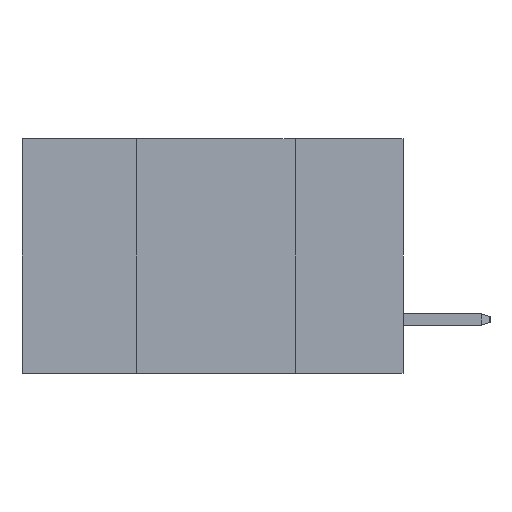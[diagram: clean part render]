
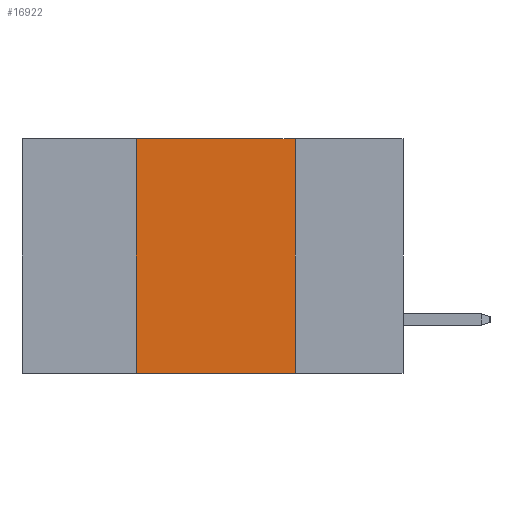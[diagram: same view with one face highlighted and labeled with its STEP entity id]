
A CAD part, left-side view. The second image highlights one B-rep face of the part: STEP entity #16922.
In plain terms, the highlighted planar face has unit normal (-1, 0, 0).
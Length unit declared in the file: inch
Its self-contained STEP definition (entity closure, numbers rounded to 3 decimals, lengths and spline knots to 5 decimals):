
#703 = CARTESIAN_POINT ( 'NONE',  ( 0., 0.42, -0.37 ) ) ;
#1049 = LINE ( 'NONE', #22835, #8461 ) ;
#1106 = LINE ( 'NONE', #4960, #2140 ) ;
#1616 = EDGE_CURVE ( 'NONE', #22002, #8231, #1049, .T. ) ;
#2140 = VECTOR ( 'NONE', #11341, 39.37008 ) ;
#2306 = ORIENTED_EDGE ( 'NONE', *, *, #1616, .F. ) ;
#2631 = EDGE_CURVE ( 'NONE', #6597, #22002, #1106, .T. ) ;
#3078 = VECTOR ( 'NONE', #9740, 39.37008 ) ;
#3267 = CARTESIAN_POINT ( 'NONE',  ( 0., 0.42, 0. ) ) ;
#4795 = ORIENTED_EDGE ( 'NONE', *, *, #22974, .T. ) ;
#4960 = CARTESIAN_POINT ( 'NONE',  ( 0., 0.6, 0. ) ) ;
#5110 = VECTOR ( 'NONE', #12046, 39.37008 ) ;
#5680 = PLANE ( 'NONE',  #6244 ) ;
#6244 = AXIS2_PLACEMENT_3D ( 'NONE', #11934, #25717, #17767 ) ;
#6597 = VERTEX_POINT ( 'NONE', #3267 ) ;
#7059 = EDGE_CURVE ( 'NONE', #12555, #6597, #21308, .T. ) ;
#7912 = CARTESIAN_POINT ( 'NONE',  ( 0., 0.6, -0.37 ) ) ;
#8231 = VERTEX_POINT ( 'NONE', #11327 ) ;
#8461 = VECTOR ( 'NONE', #13016, 39.37008 ) ;
#9740 = DIRECTION ( 'NONE',  ( 0., 0., 1. ) ) ;
#9904 = LINE ( 'NONE', #7912, #5110 ) ;
#11327 = CARTESIAN_POINT ( 'NONE',  ( 0., 0.17, -0.37 ) ) ;
#11341 = DIRECTION ( 'NONE',  ( 0., -1., 0. ) ) ;
#11668 = FACE_OUTER_BOUND ( 'NONE', #25235, .T. ) ;
#11934 = CARTESIAN_POINT ( 'NONE',  ( 0., 0.6, 0. ) ) ;
#12046 = DIRECTION ( 'NONE',  ( 0., -1., 0. ) ) ;
#12555 = VERTEX_POINT ( 'NONE', #703 ) ;
#13016 = DIRECTION ( 'NONE',  ( 0., 0., -1. ) ) ;
#14434 = ORIENTED_EDGE ( 'NONE', *, *, #2631, .F. ) ;
#16922 = ADVANCED_FACE ( 'NONE', ( #11668 ), #5680, .F. ) ;
#17084 = CARTESIAN_POINT ( 'NONE',  ( 0., 0.17, 0. ) ) ;
#17092 = ORIENTED_EDGE ( 'NONE', *, *, #7059, .F. ) ;
#17465 = CARTESIAN_POINT ( 'NONE',  ( 0., 0.42, 0. ) ) ;
#17767 = DIRECTION ( 'NONE',  ( 0., 0., -1. ) ) ;
#21308 = LINE ( 'NONE', #17465, #3078 ) ;
#22002 = VERTEX_POINT ( 'NONE', #17084 ) ;
#22835 = CARTESIAN_POINT ( 'NONE',  ( 0., 0.17, 0. ) ) ;
#22974 = EDGE_CURVE ( 'NONE', #12555, #8231, #9904, .T. ) ;
#25235 = EDGE_LOOP ( 'NONE', ( #2306, #14434, #17092, #4795 ) ) ;
#25717 = DIRECTION ( 'NONE',  ( 1., 0., 0. ) ) ;
